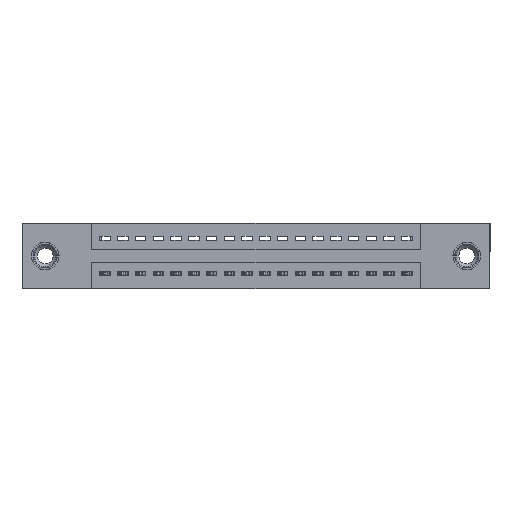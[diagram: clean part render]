
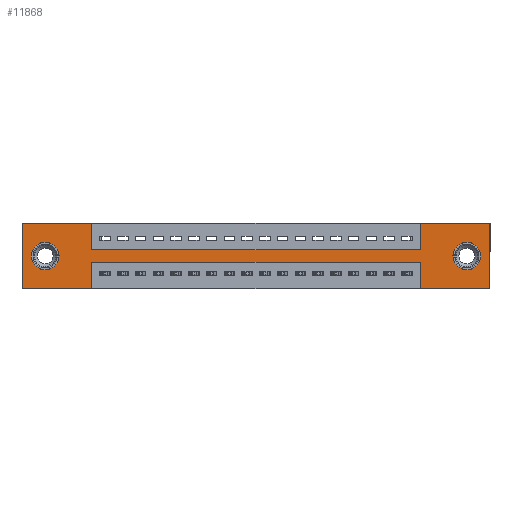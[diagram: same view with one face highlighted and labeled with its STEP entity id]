
A CAD part, front view. The second image highlights one B-rep face of the part: STEP entity #11868.
In plain terms, the highlighted planar face has unit normal (0, -1, 0).
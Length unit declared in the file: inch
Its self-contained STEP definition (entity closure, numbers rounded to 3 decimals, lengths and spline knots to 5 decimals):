
#19 = EDGE_CURVE ( 'NONE', #12360, #5412, #2754, .T. ) ;
#87 = ORIENTED_EDGE ( 'NONE', *, *, #19, .T. ) ;
#129 = CARTESIAN_POINT ( 'NONE',  ( 0.13, 0., -0.107 ) ) ;
#161 = ORIENTED_EDGE ( 'NONE', *, *, #5251, .T. ) ;
#251 = DIRECTION ( 'NONE',  ( 0., 0., 1. ) ) ;
#289 = CARTESIAN_POINT ( 'NONE',  ( 0., 0., -0.37 ) ) ;
#333 = VERTEX_POINT ( 'NONE', #9064 ) ;
#914 = DIRECTION ( 'NONE',  ( 0., 0., 1. ) ) ;
#956 = CARTESIAN_POINT ( 'NONE',  ( 2.505, 0., -0.185 ) ) ;
#1075 = VERTEX_POINT ( 'NONE', #8292 ) ;
#1100 = DIRECTION ( 'NONE',  ( 0., 1., 0. ) ) ;
#1136 = CARTESIAN_POINT ( 'NONE',  ( 2.635, 0., 0. ) ) ;
#1236 = LINE ( 'NONE', #2594, #16297 ) ;
#1283 = CARTESIAN_POINT ( 'NONE',  ( 2.635, 0., 0. ) ) ;
#1302 = EDGE_CURVE ( 'NONE', #5837, #333, #2737, .T. ) ;
#1480 = VERTEX_POINT ( 'NONE', #11935 ) ;
#1617 = EDGE_CURVE ( 'NONE', #4417, #18080, #3417, .T. ) ;
#1620 = EDGE_LOOP ( 'NONE', ( #87, #161 ) ) ;
#1801 = ORIENTED_EDGE ( 'NONE', *, *, #18684, .F. ) ;
#1840 = AXIS2_PLACEMENT_3D ( 'NONE', #18669, #1100, #9912 ) ;
#1918 = DIRECTION ( 'NONE',  ( 1., 0., 0. ) ) ;
#2002 = DIRECTION ( 'NONE',  ( 0., 0., -1. ) ) ;
#2328 = DIRECTION ( 'NONE',  ( 0., 0., -1. ) ) ;
#2546 = DIRECTION ( 'NONE',  ( -1., 0., 0. ) ) ;
#2577 = EDGE_CURVE ( 'NONE', #9730, #9419, #8728, .T. ) ;
#2594 = CARTESIAN_POINT ( 'NONE',  ( 0., 0., 0. ) ) ;
#2663 = DIRECTION ( 'NONE',  ( 0., 0., 1. ) ) ;
#2737 = LINE ( 'NONE', #7242, #8462 ) ;
#2754 = CIRCLE ( 'NONE', #1840, 0.078 ) ;
#2783 = ORIENTED_EDGE ( 'NONE', *, *, #14524, .F. ) ;
#2972 = EDGE_LOOP ( 'NONE', ( #3056, #11228, #15211, #1801, #6974, #8816, #2783, #4979, #18770, #13309, #4785, #14319 ) ) ;
#3054 = EDGE_CURVE ( 'NONE', #6478, #4417, #18230, .T. ) ;
#3056 = ORIENTED_EDGE ( 'NONE', *, *, #8783, .F. ) ;
#3417 = LINE ( 'NONE', #9078, #15066 ) ;
#3767 = EDGE_CURVE ( 'NONE', #4456, #13641, #12354, .T. ) ;
#3783 = CARTESIAN_POINT ( 'NONE',  ( 0.13, 0., -0.185 ) ) ;
#4321 = CARTESIAN_POINT ( 'NONE',  ( 2.2425, 0., 0. ) ) ;
#4397 = CARTESIAN_POINT ( 'NONE',  ( 2.2425, 0., 0. ) ) ;
#4417 = VERTEX_POINT ( 'NONE', #8636 ) ;
#4456 = VERTEX_POINT ( 'NONE', #14811 ) ;
#4587 = CARTESIAN_POINT ( 'NONE',  ( 2.2425, 0., -0.37 ) ) ;
#4667 = CARTESIAN_POINT ( 'NONE',  ( 0.13, 0., -0.263 ) ) ;
#4715 = VERTEX_POINT ( 'NONE', #5872 ) ;
#4785 = ORIENTED_EDGE ( 'NONE', *, *, #1302, .F. ) ;
#4953 = CIRCLE ( 'NONE', #13020, 0.078 ) ;
#4979 = ORIENTED_EDGE ( 'NONE', *, *, #1617, .F. ) ;
#5034 = CARTESIAN_POINT ( 'NONE',  ( 2.2425, 0., -0.15 ) ) ;
#5183 = DIRECTION ( 'NONE',  ( 0., 1., 0. ) ) ;
#5251 = EDGE_CURVE ( 'NONE', #5412, #12360, #4953, .T. ) ;
#5286 = VECTOR ( 'NONE', #2002, 39.37008 ) ;
#5412 = VERTEX_POINT ( 'NONE', #4667 ) ;
#5778 = ORIENTED_EDGE ( 'NONE', *, *, #16841, .T. ) ;
#5837 = VERTEX_POINT ( 'NONE', #6957 ) ;
#5872 = CARTESIAN_POINT ( 'NONE',  ( 0.3925, 0., -0.22 ) ) ;
#6336 = CARTESIAN_POINT ( 'NONE',  ( 0.3925, 0., -0.37 ) ) ;
#6478 = VERTEX_POINT ( 'NONE', #6820 ) ;
#6507 = FACE_BOUND ( 'NONE', #1620, .T. ) ;
#6793 = EDGE_CURVE ( 'NONE', #333, #6478, #1236, .T. ) ;
#6820 = CARTESIAN_POINT ( 'NONE',  ( 0.3925, 0., 0. ) ) ;
#6957 = CARTESIAN_POINT ( 'NONE',  ( 0., 0., -0.37 ) ) ;
#6974 = ORIENTED_EDGE ( 'NONE', *, *, #8376, .F. ) ;
#7220 = CARTESIAN_POINT ( 'NONE',  ( 0., 0., 0. ) ) ;
#7242 = CARTESIAN_POINT ( 'NONE',  ( 0., 0., 0. ) ) ;
#7582 = AXIS2_PLACEMENT_3D ( 'NONE', #289, #10529, #13478 ) ;
#7837 = VECTOR ( 'NONE', #10856, 39.37008 ) ;
#8292 = CARTESIAN_POINT ( 'NONE',  ( 2.635, 0., -0.37 ) ) ;
#8376 = EDGE_CURVE ( 'NONE', #9419, #1075, #9442, .T. ) ;
#8462 = VECTOR ( 'NONE', #11793, 39.37008 ) ;
#8482 = EDGE_CURVE ( 'NONE', #11998, #5837, #11708, .T. ) ;
#8636 = CARTESIAN_POINT ( 'NONE',  ( 0.3925, 0., -0.15 ) ) ;
#8728 = LINE ( 'NONE', #7220, #18328 ) ;
#8783 = EDGE_CURVE ( 'NONE', #4715, #11998, #16931, .T. ) ;
#8816 = ORIENTED_EDGE ( 'NONE', *, *, #2577, .F. ) ;
#9036 = CIRCLE ( 'NONE', #13536, 0.078 ) ;
#9064 = CARTESIAN_POINT ( 'NONE',  ( 0., 0., 0. ) ) ;
#9078 = CARTESIAN_POINT ( 'NONE',  ( 0.3925, 0., -0.15 ) ) ;
#9159 = CARTESIAN_POINT ( 'NONE',  ( 0.3925, 0., 0. ) ) ;
#9419 = VERTEX_POINT ( 'NONE', #1136 ) ;
#9442 = LINE ( 'NONE', #1283, #16733 ) ;
#9730 = VERTEX_POINT ( 'NONE', #4321 ) ;
#9912 = DIRECTION ( 'NONE',  ( 0., 0., 1. ) ) ;
#10017 = VECTOR ( 'NONE', #11860, 39.37008 ) ;
#10529 = DIRECTION ( 'NONE',  ( 0., -1., 0. ) ) ;
#10557 = LINE ( 'NONE', #4397, #17823 ) ;
#10836 = VECTOR ( 'NONE', #2546, 39.37008 ) ;
#10856 = DIRECTION ( 'NONE',  ( -1., 0., 0. ) ) ;
#11228 = ORIENTED_EDGE ( 'NONE', *, *, #13338, .F. ) ;
#11708 = LINE ( 'NONE', #16445, #18341 ) ;
#11793 = DIRECTION ( 'NONE',  ( 0., 0., 1. ) ) ;
#11860 = DIRECTION ( 'NONE',  ( 0., 0., -1. ) ) ;
#11868 = ADVANCED_FACE ( 'NONE', ( #12249, #6507, #14741 ), #16493, .T. ) ;
#11935 = CARTESIAN_POINT ( 'NONE',  ( 2.2425, 0., -0.22 ) ) ;
#11998 = VERTEX_POINT ( 'NONE', #13186 ) ;
#12249 = FACE_BOUND ( 'NONE', #12943, .T. ) ;
#12354 = CIRCLE ( 'NONE', #12837, 0.078 ) ;
#12360 = VERTEX_POINT ( 'NONE', #129 ) ;
#12581 = DIRECTION ( 'NONE',  ( 0., 1., 0. ) ) ;
#12725 = DIRECTION ( 'NONE',  ( 0., 0., -1. ) ) ;
#12837 = AXIS2_PLACEMENT_3D ( 'NONE', #956, #14282, #12725 ) ;
#12943 = EDGE_LOOP ( 'NONE', ( #16731, #5778 ) ) ;
#13020 = AXIS2_PLACEMENT_3D ( 'NONE', #3783, #5183, #914 ) ;
#13186 = CARTESIAN_POINT ( 'NONE',  ( 0.3925, 0., -0.37 ) ) ;
#13309 = ORIENTED_EDGE ( 'NONE', *, *, #6793, .F. ) ;
#13338 = EDGE_CURVE ( 'NONE', #1480, #4715, #17416, .T. ) ;
#13478 = DIRECTION ( 'NONE',  ( 0., 0., -1. ) ) ;
#13536 = AXIS2_PLACEMENT_3D ( 'NONE', #15361, #12581, #2328 ) ;
#13641 = VERTEX_POINT ( 'NONE', #17616 ) ;
#13981 = EDGE_CURVE ( 'NONE', #17859, #1480, #14887, .T. ) ;
#14282 = DIRECTION ( 'NONE',  ( 0., 1., 0. ) ) ;
#14319 = ORIENTED_EDGE ( 'NONE', *, *, #8482, .F. ) ;
#14524 = EDGE_CURVE ( 'NONE', #18080, #9730, #10557, .T. ) ;
#14741 = FACE_OUTER_BOUND ( 'NONE', #2972, .T. ) ;
#14811 = CARTESIAN_POINT ( 'NONE',  ( 2.505, 0., -0.107 ) ) ;
#14887 = LINE ( 'NONE', #4587, #16939 ) ;
#15066 = VECTOR ( 'NONE', #1918, 39.37008 ) ;
#15211 = ORIENTED_EDGE ( 'NONE', *, *, #13981, .F. ) ;
#15361 = CARTESIAN_POINT ( 'NONE',  ( 2.505, 0., -0.185 ) ) ;
#16174 = DIRECTION ( 'NONE',  ( 1., 0., 0. ) ) ;
#16297 = VECTOR ( 'NONE', #16174, 39.37008 ) ;
#16445 = CARTESIAN_POINT ( 'NONE',  ( 0., 0., -0.37 ) ) ;
#16493 = PLANE ( 'NONE',  #7582 ) ;
#16509 = DIRECTION ( 'NONE',  ( -1., 0., 0. ) ) ;
#16513 = CARTESIAN_POINT ( 'NONE',  ( 2.2425, 0., -0.37 ) ) ;
#16620 = CARTESIAN_POINT ( 'NONE',  ( 0., 0., -0.37 ) ) ;
#16731 = ORIENTED_EDGE ( 'NONE', *, *, #3767, .T. ) ;
#16733 = VECTOR ( 'NONE', #17402, 39.37008 ) ;
#16841 = EDGE_CURVE ( 'NONE', #13641, #4456, #9036, .T. ) ;
#16931 = LINE ( 'NONE', #6336, #5286 ) ;
#16939 = VECTOR ( 'NONE', #251, 39.37008 ) ;
#16958 = LINE ( 'NONE', #16620, #7837 ) ;
#17402 = DIRECTION ( 'NONE',  ( 0., 0., -1. ) ) ;
#17416 = LINE ( 'NONE', #18519, #10836 ) ;
#17616 = CARTESIAN_POINT ( 'NONE',  ( 2.505, 0., -0.263 ) ) ;
#17823 = VECTOR ( 'NONE', #2663, 39.37008 ) ;
#17859 = VERTEX_POINT ( 'NONE', #16513 ) ;
#18080 = VERTEX_POINT ( 'NONE', #5034 ) ;
#18230 = LINE ( 'NONE', #9159, #10017 ) ;
#18328 = VECTOR ( 'NONE', #18939, 39.37008 ) ;
#18341 = VECTOR ( 'NONE', #16509, 39.37008 ) ;
#18519 = CARTESIAN_POINT ( 'NONE',  ( 0.3925, 0., -0.22 ) ) ;
#18669 = CARTESIAN_POINT ( 'NONE',  ( 0.13, 0., -0.185 ) ) ;
#18684 = EDGE_CURVE ( 'NONE', #1075, #17859, #16958, .T. ) ;
#18770 = ORIENTED_EDGE ( 'NONE', *, *, #3054, .F. ) ;
#18939 = DIRECTION ( 'NONE',  ( 1., 0., 0. ) ) ;
